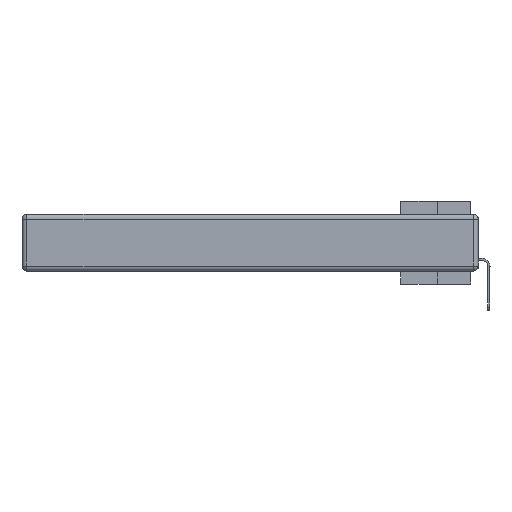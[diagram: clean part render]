
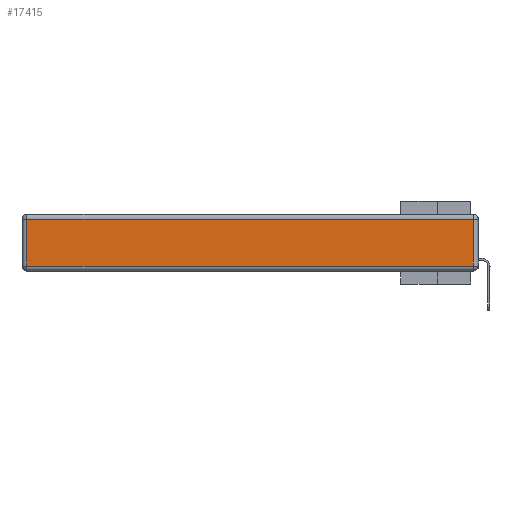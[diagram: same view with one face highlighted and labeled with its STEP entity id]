
A CAD part, left-side view. The second image highlights one B-rep face of the part: STEP entity #17415.
In plain terms, the highlighted planar face has unit normal (-1, 0, 0).
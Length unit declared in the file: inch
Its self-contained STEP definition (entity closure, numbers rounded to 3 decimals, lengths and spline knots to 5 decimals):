
#186 = LINE ( 'NONE', #15137, #1954 ) ;
#1113 = EDGE_CURVE ( 'NONE', #23544, #23552, #6449, .T. ) ;
#1954 = VECTOR ( 'NONE', #26558, 39.37008 ) ;
#1960 = CARTESIAN_POINT ( 'NONE',  ( 0., 2.75, -0.03 ) ) ;
#2156 = CARTESIAN_POINT ( 'NONE',  ( 0., 2.72, -0.03 ) ) ;
#2763 = VECTOR ( 'NONE', #4324, 39.37008 ) ;
#4324 = DIRECTION ( 'NONE',  ( 0., 1., 0. ) ) ;
#5339 = ORIENTED_EDGE ( 'NONE', *, *, #18271, .T. ) ;
#6082 = VERTEX_POINT ( 'NONE', #20888 ) ;
#6262 = EDGE_CURVE ( 'NONE', #29736, #23544, #9267, .T. ) ;
#6449 = LINE ( 'NONE', #12154, #8881 ) ;
#8881 = VECTOR ( 'NONE', #15501, 39.37008 ) ;
#9267 = LINE ( 'NONE', #18723, #35065 ) ;
#12154 = CARTESIAN_POINT ( 'NONE',  ( 0., 0., -0.313 ) ) ;
#14353 = ORIENTED_EDGE ( 'NONE', *, *, #30957, .T. ) ;
#14642 = AXIS2_PLACEMENT_3D ( 'NONE', #27651, #34504, #19761 ) ;
#15137 = CARTESIAN_POINT ( 'NONE',  ( 0., 0.03, -0.343 ) ) ;
#15501 = DIRECTION ( 'NONE',  ( 0., -1., 0. ) ) ;
#16911 = LINE ( 'NONE', #1960, #2763 ) ;
#17415 = ADVANCED_FACE ( 'NONE', ( #28221 ), #18607, .T. ) ;
#18271 = EDGE_CURVE ( 'NONE', #6082, #29736, #16911, .T. ) ;
#18607 = PLANE ( 'NONE',  #14642 ) ;
#18723 = CARTESIAN_POINT ( 'NONE',  ( 0., 2.72, -0.343 ) ) ;
#19761 = DIRECTION ( 'NONE',  ( 0., 0., 1. ) ) ;
#20888 = CARTESIAN_POINT ( 'NONE',  ( 0., 0.03, -0.03 ) ) ;
#23544 = VERTEX_POINT ( 'NONE', #26412 ) ;
#23552 = VERTEX_POINT ( 'NONE', #31722 ) ;
#26412 = CARTESIAN_POINT ( 'NONE',  ( 0., 2.72, -0.313 ) ) ;
#26558 = DIRECTION ( 'NONE',  ( 0., 0., 1. ) ) ;
#27651 = CARTESIAN_POINT ( 'NONE',  ( 0., 0., -0.343 ) ) ;
#27759 = ORIENTED_EDGE ( 'NONE', *, *, #1113, .T. ) ;
#27957 = DIRECTION ( 'NONE',  ( 0., 0., -1. ) ) ;
#28221 = FACE_OUTER_BOUND ( 'NONE', #35387, .T. ) ;
#28269 = ORIENTED_EDGE ( 'NONE', *, *, #6262, .T. ) ;
#29736 = VERTEX_POINT ( 'NONE', #2156 ) ;
#30957 = EDGE_CURVE ( 'NONE', #23552, #6082, #186, .T. ) ;
#31722 = CARTESIAN_POINT ( 'NONE',  ( 0., 0.03, -0.313 ) ) ;
#34504 = DIRECTION ( 'NONE',  ( -1., 0., 0. ) ) ;
#35065 = VECTOR ( 'NONE', #27957, 39.37008 ) ;
#35387 = EDGE_LOOP ( 'NONE', ( #27759, #14353, #5339, #28269 ) ) ;
